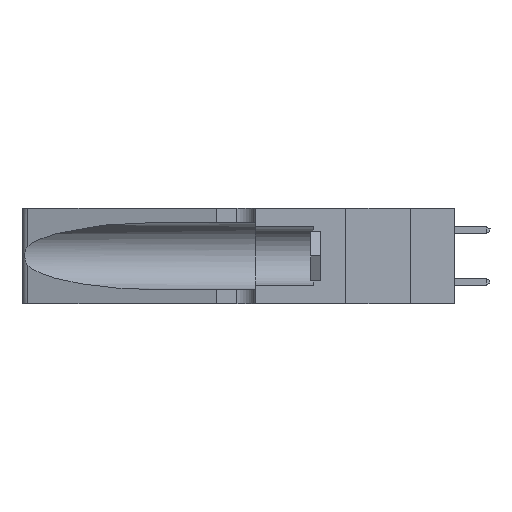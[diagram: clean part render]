
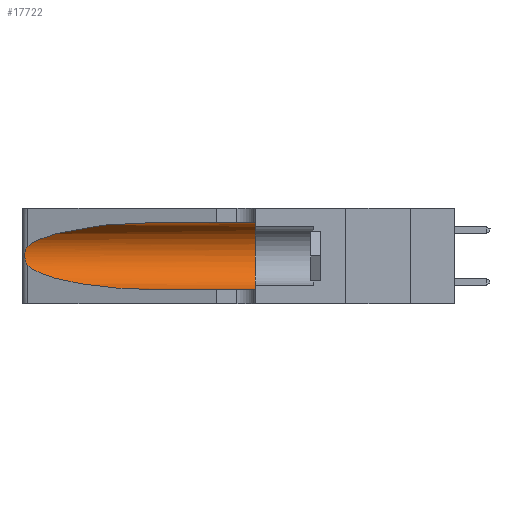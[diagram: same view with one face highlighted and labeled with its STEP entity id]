
A CAD part, left-side view. The second image highlights one B-rep face of the part: STEP entity #17722.
In plain terms, the highlighted cylindrical face has radius 3.308 mm (diameter 6.617 mm), a partial arc.
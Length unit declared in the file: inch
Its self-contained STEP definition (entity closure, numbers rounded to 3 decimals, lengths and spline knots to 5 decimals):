
#607 = CARTESIAN_POINT ( 'NONE',  ( 0.1305, 1.61858, 0.185 ) ) ;
#784 = CARTESIAN_POINT ( 'NONE',  ( 0.25854, 1.2359, 0.20912 ) ) ;
#922 = CARTESIAN_POINT ( 'NONE',  ( 0.25787, 1.23484, 0.2124 ) ) ;
#1798 = VERTEX_POINT ( 'NONE', #25932 ) ;
#2170 = CARTESIAN_POINT ( 'NONE',  ( 0.2373, 1.15595, 0.08982 ) ) ;
#2375 = ORIENTED_EDGE ( 'NONE', *, *, #34410, .T. ) ;
#3425 = DIRECTION ( 'NONE',  ( 0., -1., 0. ) ) ;
#3941 = CARTESIAN_POINT ( 'NONE',  ( 0.26075, 1.23896, 0.19203 ) ) ;
#4195 = CARTESIAN_POINT ( 'NONE',  ( 0.26018, 1.23835, 0.19895 ) ) ;
#4331 = CARTESIAN_POINT ( 'NONE',  ( 0.25555, 1.22993, 0.14849 ) ) ;
#4761 = CARTESIAN_POINT ( 'NONE',  ( 0.25487, 1.22718, 0.22369 ) ) ;
#4874 = VERTEX_POINT ( 'NONE', #37356 ) ;
#6047 = CARTESIAN_POINT ( 'NONE',  ( 0.1305, 1.61858, 0.05475 ) ) ;
#7050 = EDGE_CURVE ( 'NONE', #10763, #11075, #31913, .T. ) ;
#7219 = CARTESIAN_POINT ( 'NONE',  ( 0.1305, 0.72297, 0.31525 ) ) ;
#7530 = CARTESIAN_POINT ( 'NONE',  ( 0.25487, 1.22718, 0.22369 ) ) ;
#7805 =( BOUNDED_CURVE ( )  B_SPLINE_CURVE ( 3, ( #28488, #2170, #37935, #28619 ),
 .UNSPECIFIED., .F., .T. ) 
 B_SPLINE_CURVE_WITH_KNOTS ( ( 4, 4 ),
 ( 3.44316, 4.71239 ),
 .UNSPECIFIED. ) 
 CURVE ( )  GEOMETRIC_REPRESENTATION_ITEM ( )  RATIONAL_B_SPLINE_CURVE ( ( 1., 0.87, 0.87, 1. ) ) 
 REPRESENTATION_ITEM ( '' )  );
#8069 = CARTESIAN_POINT ( 'NONE',  ( 0.1305, 0.72297, 0.31525 ) ) ;
#8345 = EDGE_LOOP ( 'NONE', ( #14254, #20929, #31615, #2375, #35353, #14201 ) ) ;
#9054 = AXIS2_PLACEMENT_3D ( 'NONE', #9437, #12693, #30236 ) ;
#9147 = DIRECTION ( 'NONE',  ( 0., 0., -1. ) ) ;
#9437 = CARTESIAN_POINT ( 'NONE',  ( 0.1305, 0.35, 0.185 ) ) ;
#9903 = CARTESIAN_POINT ( 'NONE',  ( 0.26017, 1.23833, 0.17102 ) ) ;
#10603 = CARTESIAN_POINT ( 'NONE',  ( 0.1305, 1.61858, 0.31525 ) ) ;
#10711 = VECTOR ( 'NONE', #31124, 39.37008 ) ;
#10763 = VERTEX_POINT ( 'NONE', #8069 ) ;
#11075 = VERTEX_POINT ( 'NONE', #7530 ) ;
#12693 = DIRECTION ( 'NONE',  ( 0., 1., 0. ) ) ;
#13306 = CARTESIAN_POINT ( 'NONE',  ( 0.25487, 1.22718, 0.14631 ) ) ;
#13904 = LINE ( 'NONE', #6047, #36673 ) ;
#14201 = ORIENTED_EDGE ( 'NONE', *, *, #26614, .F. ) ;
#14254 = ORIENTED_EDGE ( 'NONE', *, *, #7050, .T. ) ;
#16568 = EDGE_CURVE ( 'NONE', #4874, #1798, #21194, .T. ) ;
#17722 = ADVANCED_FACE ( 'NONE', ( #23548 ), #20757, .F. ) ;
#18139 = LINE ( 'NONE', #10603, #10711 ) ;
#18626 = CARTESIAN_POINT ( 'NONE',  ( 0.25487, 1.22718, 0.22369 ) ) ;
#18749 = CARTESIAN_POINT ( 'NONE',  ( 0.25639, 1.23184, 0.21858 ) ) ;
#19268 = CARTESIAN_POINT ( 'NONE',  ( 0.25639, 1.23186, 0.15144 ) ) ;
#19580 = CARTESIAN_POINT ( 'NONE',  ( 0.2373, 1.15595, 0.28018 ) ) ;
#20052 = VERTEX_POINT ( 'NONE', #33253 ) ;
#20757 = CYLINDRICAL_SURFACE ( 'NONE', #27950, 0.13025 ) ;
#20929 = ORIENTED_EDGE ( 'NONE', *, *, #32665, .T. ) ;
#21194 = CIRCLE ( 'NONE', #9054, 0.13025 ) ;
#21594 = EDGE_CURVE ( 'NONE', #28527, #20052, #7805, .T. ) ;
#21975 = CARTESIAN_POINT ( 'NONE',  ( 0.25555, 1.22994, 0.2215 ) ) ;
#22417 = CARTESIAN_POINT ( 'NONE',  ( 0.18966, 0.96281, 0.31525 ) ) ;
#23548 = FACE_OUTER_BOUND ( 'NONE', #8345, .T. ) ;
#24699 = CARTESIAN_POINT ( 'NONE',  ( 0.26075, 1.23896, 0.178 ) ) ;
#24961 = CARTESIAN_POINT ( 'NONE',  ( 0.25856, 1.23593, 0.16098 ) ) ;
#25932 = CARTESIAN_POINT ( 'NONE',  ( 0.1305, 0.35, 0.05475 ) ) ;
#26614 = EDGE_CURVE ( 'NONE', #10763, #4874, #18139, .T. ) ;
#27818 = CARTESIAN_POINT ( 'NONE',  ( 0.25487, 1.22718, 0.14631 ) ) ;
#27950 = AXIS2_PLACEMENT_3D ( 'NONE', #607, #3425, #9147 ) ;
#28488 = CARTESIAN_POINT ( 'NONE',  ( 0.25487, 1.22718, 0.14631 ) ) ;
#28527 = VERTEX_POINT ( 'NONE', #27818 ) ;
#28619 = CARTESIAN_POINT ( 'NONE',  ( 0.1305, 0.72297, 0.05475 ) ) ;
#30236 = DIRECTION ( 'NONE',  ( 0., 0., 1. ) ) ;
#31124 = DIRECTION ( 'NONE',  ( 0., -1., 0. ) ) ;
#31615 = ORIENTED_EDGE ( 'NONE', *, *, #21594, .T. ) ;
#31913 =( BOUNDED_CURVE ( )  B_SPLINE_CURVE ( 3, ( #7219, #22417, #19580, #4761 ),
 .UNSPECIFIED., .F., .T. ) 
 B_SPLINE_CURVE_WITH_KNOTS ( ( 4, 4 ),
 ( 1.5708, 2.84003 ),
 .UNSPECIFIED. ) 
 CURVE ( )  GEOMETRIC_REPRESENTATION_ITEM ( )  RATIONAL_B_SPLINE_CURVE ( ( 1., 0.87, 0.87, 1. ) ) 
 REPRESENTATION_ITEM ( '' )  );
#32665 = EDGE_CURVE ( 'NONE', #11075, #28527, #35956, .T. ) ;
#33253 = CARTESIAN_POINT ( 'NONE',  ( 0.1305, 0.72297, 0.05475 ) ) ;
#34410 = EDGE_CURVE ( 'NONE', #20052, #1798, #13904, .T. ) ;
#35353 = ORIENTED_EDGE ( 'NONE', *, *, #16568, .F. ) ;
#35685 = DIRECTION ( 'NONE',  ( 0., -1., 0. ) ) ;
#35956 = B_SPLINE_CURVE_WITH_KNOTS ( 'NONE', 3,
 ( #18626, #21975, #18749, #922, #784, #4195, #3941, #24699, #9903, #24961, #37096, #19268, #4331, #13306 ),
 .UNSPECIFIED., .F., .F.,
 ( 4, 2, 2, 2, 2, 2, 4 ),
 ( 0., 0.00027, 0.00053, 0.00107, 0.0016, 0.00187, 0.00214 ),
 .UNSPECIFIED. ) ;
#36673 = VECTOR ( 'NONE', #35685, 39.37008 ) ;
#37096 = CARTESIAN_POINT ( 'NONE',  ( 0.25789, 1.23486, 0.15765 ) ) ;
#37356 = CARTESIAN_POINT ( 'NONE',  ( 0.1305, 0.35, 0.31525 ) ) ;
#37935 = CARTESIAN_POINT ( 'NONE',  ( 0.18966, 0.96281, 0.05475 ) ) ;
